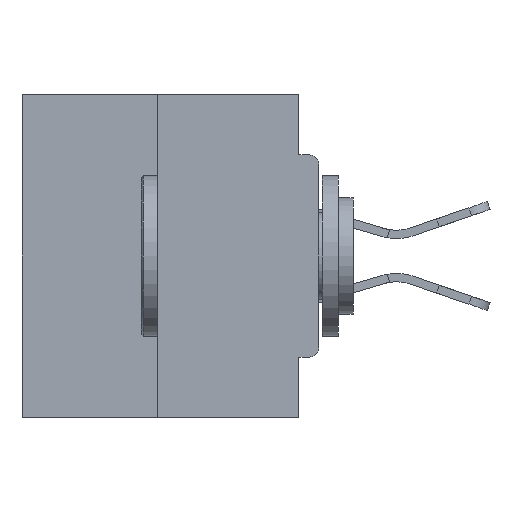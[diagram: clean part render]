
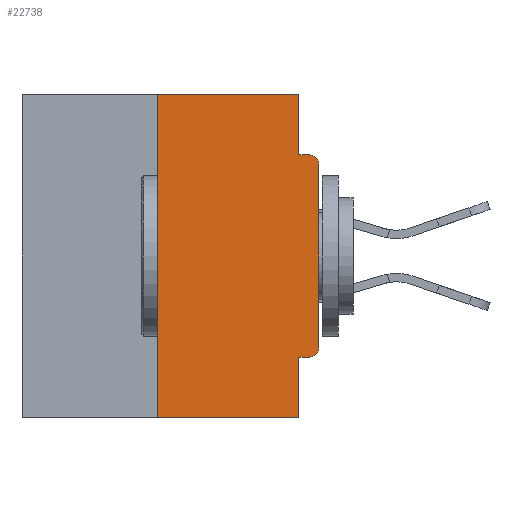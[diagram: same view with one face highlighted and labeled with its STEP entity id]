
A CAD part, left-side view. The second image highlights one B-rep face of the part: STEP entity #22738.
In plain terms, the highlighted planar face has unit normal (-1, 0, 0).
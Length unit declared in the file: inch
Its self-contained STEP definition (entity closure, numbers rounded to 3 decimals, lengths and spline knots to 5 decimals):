
#890 = VECTOR ( 'NONE', #22462, 39.37008 ) ;
#1231 = CARTESIAN_POINT ( 'NONE',  ( 0., 0.031, -0.5 ) ) ;
#1238 = CARTESIAN_POINT ( 'NONE',  ( 0., 0.031, 0. ) ) ;
#1346 = CARTESIAN_POINT ( 'NONE',  ( 0., 0., -0.3915 ) ) ;
#1434 = VERTEX_POINT ( 'NONE', #21155 ) ;
#1555 = DIRECTION ( 'NONE',  ( -1., 0., 0. ) ) ;
#1687 = DIRECTION ( 'NONE',  ( 0., 0., -1. ) ) ;
#1743 = VECTOR ( 'NONE', #28549, 39.37008 ) ;
#2215 = DIRECTION ( 'NONE',  ( 0., 0., 1. ) ) ;
#2426 = EDGE_CURVE ( 'NONE', #22961, #11850, #33279, .T. ) ;
#2690 = CARTESIAN_POINT ( 'NONE',  ( 0., 0.25, 0. ) ) ;
#3795 = CARTESIAN_POINT ( 'NONE',  ( 0., 0.46, 0. ) ) ;
#3814 = DIRECTION ( 'NONE',  ( 0., 0., 1. ) ) ;
#3918 = CARTESIAN_POINT ( 'NONE',  ( 0., 0.25, 0. ) ) ;
#4022 = ORIENTED_EDGE ( 'NONE', *, *, #22977, .T. ) ;
#4636 = EDGE_CURVE ( 'NONE', #24932, #7149, #6058, .T. ) ;
#5424 = CARTESIAN_POINT ( 'NONE',  ( 0., 0., -0.1085 ) ) ;
#5844 = ORIENTED_EDGE ( 'NONE', *, *, #10126, .F. ) ;
#6042 = AXIS2_PLACEMENT_3D ( 'NONE', #3795, #20257, #19393 ) ;
#6058 = LINE ( 'NONE', #12356, #1743 ) ;
#6128 = ORIENTED_EDGE ( 'NONE', *, *, #11531, .T. ) ;
#7149 = VERTEX_POINT ( 'NONE', #1231 ) ;
#7593 = VECTOR ( 'NONE', #29003, 39.37008 ) ;
#8460 = DIRECTION ( 'NONE',  ( 0., -1., 0. ) ) ;
#8532 = EDGE_CURVE ( 'NONE', #31211, #7149, #11886, .T. ) ;
#9563 = ORIENTED_EDGE ( 'NONE', *, *, #22226, .F. ) ;
#10126 = EDGE_CURVE ( 'NONE', #11850, #10857, #16146, .T. ) ;
#10666 = ORIENTED_EDGE ( 'NONE', *, *, #4636, .T. ) ;
#10857 = VERTEX_POINT ( 'NONE', #28750 ) ;
#11531 = EDGE_CURVE ( 'NONE', #32161, #21372, #31521, .T. ) ;
#11850 = VERTEX_POINT ( 'NONE', #14445 ) ;
#11886 = LINE ( 'NONE', #33892, #20882 ) ;
#12039 = VECTOR ( 'NONE', #12902, 39.37008 ) ;
#12356 = CARTESIAN_POINT ( 'NONE',  ( 0., 0.46, -0.5 ) ) ;
#12902 = DIRECTION ( 'NONE',  ( 0., -1., 0. ) ) ;
#12928 = ORIENTED_EDGE ( 'NONE', *, *, #13558, .T. ) ;
#13558 = EDGE_CURVE ( 'NONE', #21372, #1434, #23199, .T. ) ;
#13883 = CARTESIAN_POINT ( 'NONE',  ( 0., 0.46, 0. ) ) ;
#14093 = ORIENTED_EDGE ( 'NONE', *, *, #8532, .F. ) ;
#14223 = FACE_OUTER_BOUND ( 'NONE', #23728, .T. ) ;
#14445 = CARTESIAN_POINT ( 'NONE',  ( 0., 0.031, 0. ) ) ;
#15133 = LINE ( 'NONE', #25120, #890 ) ;
#15307 = CARTESIAN_POINT ( 'NONE',  ( 0., 0.031, -0.4065 ) ) ;
#15540 = LINE ( 'NONE', #2690, #15973 ) ;
#15973 = VECTOR ( 'NONE', #2215, 39.37008 ) ;
#16146 = LINE ( 'NONE', #1238, #7593 ) ;
#17287 = ORIENTED_EDGE ( 'NONE', *, *, #30091, .F. ) ;
#17387 = CARTESIAN_POINT ( 'NONE',  ( 0., 0., 0. ) ) ;
#17842 = ORIENTED_EDGE ( 'NONE', *, *, #22179, .F. ) ;
#18493 = ORIENTED_EDGE ( 'NONE', *, *, #2426, .F. ) ;
#19272 = PLANE ( 'NONE',  #6042 ) ;
#19393 = DIRECTION ( 'NONE',  ( 0., 0., -1. ) ) ;
#19602 = CARTESIAN_POINT ( 'NONE',  ( 0., 0.25, -0.5 ) ) ;
#19912 = AXIS2_PLACEMENT_3D ( 'NONE', #23408, #1555, #1687 ) ;
#20257 = DIRECTION ( 'NONE',  ( 1., 0., 0. ) ) ;
#20626 = CIRCLE ( 'NONE', #25369, 0.015 ) ;
#20714 = VERTEX_POINT ( 'NONE', #34491 ) ;
#20882 = VECTOR ( 'NONE', #31360, 39.37008 ) ;
#21155 = CARTESIAN_POINT ( 'NONE',  ( 0., 0.015, -0.0935 ) ) ;
#21372 = VERTEX_POINT ( 'NONE', #5424 ) ;
#22179 = EDGE_CURVE ( 'NONE', #24932, #22961, #15540, .T. ) ;
#22226 = EDGE_CURVE ( 'NONE', #20714, #31211, #15133, .T. ) ;
#22462 = DIRECTION ( 'NONE',  ( 0., 1., 0. ) ) ;
#22738 = ADVANCED_FACE ( 'NONE', ( #14223 ), #19272, .F. ) ;
#22961 = VERTEX_POINT ( 'NONE', #3918 ) ;
#22977 = EDGE_CURVE ( 'NONE', #20714, #32161, #20626, .T. ) ;
#23199 = CIRCLE ( 'NONE', #19912, 0.015 ) ;
#23408 = CARTESIAN_POINT ( 'NONE',  ( 0., 0.015, -0.1085 ) ) ;
#23728 = EDGE_LOOP ( 'NONE', ( #18493, #17842, #10666, #14093, #9563, #4022, #6128, #12928, #17287, #5844 ) ) ;
#24020 = CARTESIAN_POINT ( 'NONE',  ( 0., 0., -0.0935 ) ) ;
#24180 = DIRECTION ( 'NONE',  ( 0., 0., -1. ) ) ;
#24932 = VERTEX_POINT ( 'NONE', #19602 ) ;
#25120 = CARTESIAN_POINT ( 'NONE',  ( 0., 0., -0.4065 ) ) ;
#25369 = AXIS2_PLACEMENT_3D ( 'NONE', #32994, #32619, #24180 ) ;
#27170 = VECTOR ( 'NONE', #3814, 39.37008 ) ;
#28549 = DIRECTION ( 'NONE',  ( 0., -1., 0. ) ) ;
#28750 = CARTESIAN_POINT ( 'NONE',  ( 0., 0.031, -0.0935 ) ) ;
#29003 = DIRECTION ( 'NONE',  ( 0., 0., -1. ) ) ;
#30091 = EDGE_CURVE ( 'NONE', #10857, #1434, #34392, .T. ) ;
#31211 = VERTEX_POINT ( 'NONE', #15307 ) ;
#31360 = DIRECTION ( 'NONE',  ( 0., 0., -1. ) ) ;
#31521 = LINE ( 'NONE', #17387, #27170 ) ;
#32161 = VERTEX_POINT ( 'NONE', #1346 ) ;
#32619 = DIRECTION ( 'NONE',  ( -1., 0., 0. ) ) ;
#32845 = VECTOR ( 'NONE', #8460, 39.37008 ) ;
#32994 = CARTESIAN_POINT ( 'NONE',  ( 0., 0.015, -0.3915 ) ) ;
#33279 = LINE ( 'NONE', #13883, #32845 ) ;
#33892 = CARTESIAN_POINT ( 'NONE',  ( 0., 0.031, -0.5 ) ) ;
#34392 = LINE ( 'NONE', #24020, #12039 ) ;
#34491 = CARTESIAN_POINT ( 'NONE',  ( 0., 0.015, -0.4065 ) ) ;
